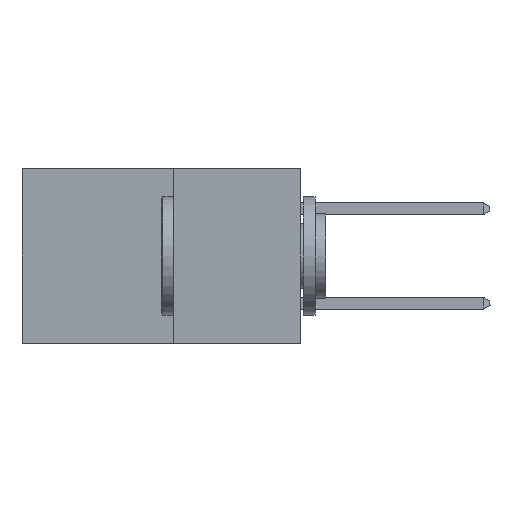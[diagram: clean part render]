
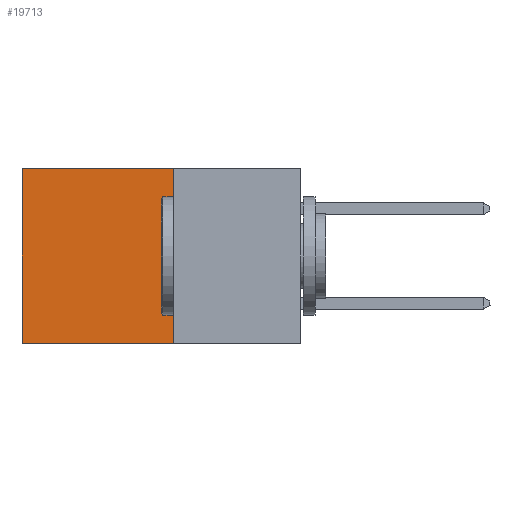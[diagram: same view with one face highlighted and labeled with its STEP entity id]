
A CAD part, left-side view. The second image highlights one B-rep face of the part: STEP entity #19713.
In plain terms, the highlighted planar face has unit normal (-1, 0, 0).
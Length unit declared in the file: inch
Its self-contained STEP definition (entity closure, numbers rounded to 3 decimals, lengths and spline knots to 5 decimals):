
#127 = LINE ( 'NONE', #739, #3368 ) ;
#260 = LINE ( 'NONE', #8819, #4022 ) ;
#739 = CARTESIAN_POINT ( 'NONE',  ( 0.277, 0.27, -0.37 ) ) ;
#1366 = CARTESIAN_POINT ( 'NONE',  ( 0.277, 0.27, -0.37 ) ) ;
#2632 = DIRECTION ( 'NONE',  ( 0., 0., -1. ) ) ;
#2988 = DIRECTION ( 'NONE',  ( 1., 0., 0. ) ) ;
#3128 = ORIENTED_EDGE ( 'NONE', *, *, #12639, .T. ) ;
#3307 = EDGE_CURVE ( 'NONE', #7169, #6030, #127, .T. ) ;
#3368 = VECTOR ( 'NONE', #2632, 39.37008 ) ;
#4022 = VECTOR ( 'NONE', #8918, 39.37008 ) ;
#4099 = CARTESIAN_POINT ( 'NONE',  ( 0.277, 0.27, 0. ) ) ;
#5433 = VERTEX_POINT ( 'NONE', #6420 ) ;
#5684 = DIRECTION ( 'NONE',  ( 0., 1., 0. ) ) ;
#5706 = CARTESIAN_POINT ( 'NONE',  ( 0.277, 0.27, 0. ) ) ;
#6030 = VERTEX_POINT ( 'NONE', #8903 ) ;
#6420 = CARTESIAN_POINT ( 'NONE',  ( 0.277, 0.59, -0.37 ) ) ;
#7169 = VERTEX_POINT ( 'NONE', #5706 ) ;
#7729 = VECTOR ( 'NONE', #5684, 39.37008 ) ;
#8227 = LINE ( 'NONE', #4099, #7729 ) ;
#8819 = CARTESIAN_POINT ( 'NONE',  ( 0.277, 0.59, -0.37 ) ) ;
#8826 = AXIS2_PLACEMENT_3D ( 'NONE', #1366, #2988, #14415 ) ;
#8833 = EDGE_CURVE ( 'NONE', #20362, #5433, #260, .T. ) ;
#8903 = CARTESIAN_POINT ( 'NONE',  ( 0.277, 0.27, -0.37 ) ) ;
#8918 = DIRECTION ( 'NONE',  ( 0., 0., -1. ) ) ;
#8957 = LINE ( 'NONE', #19545, #12907 ) ;
#11553 = DIRECTION ( 'NONE',  ( 0., 1., 0. ) ) ;
#12639 = EDGE_CURVE ( 'NONE', #7169, #20362, #8227, .T. ) ;
#12907 = VECTOR ( 'NONE', #11553, 39.37008 ) ;
#12980 = ORIENTED_EDGE ( 'NONE', *, *, #3307, .F. ) ;
#14415 = DIRECTION ( 'NONE',  ( 0., 0., -1. ) ) ;
#14828 = FACE_OUTER_BOUND ( 'NONE', #20199, .T. ) ;
#16040 = ORIENTED_EDGE ( 'NONE', *, *, #8833, .T. ) ;
#17852 = CARTESIAN_POINT ( 'NONE',  ( 0.277, 0.59, 0. ) ) ;
#18393 = EDGE_CURVE ( 'NONE', #6030, #5433, #8957, .T. ) ;
#19545 = CARTESIAN_POINT ( 'NONE',  ( 0.277, 0.27, -0.37 ) ) ;
#19713 = ADVANCED_FACE ( 'NONE', ( #14828 ), #20718, .F. ) ;
#20179 = ORIENTED_EDGE ( 'NONE', *, *, #18393, .F. ) ;
#20199 = EDGE_LOOP ( 'NONE', ( #16040, #20179, #12980, #3128 ) ) ;
#20362 = VERTEX_POINT ( 'NONE', #17852 ) ;
#20718 = PLANE ( 'NONE',  #8826 ) ;
